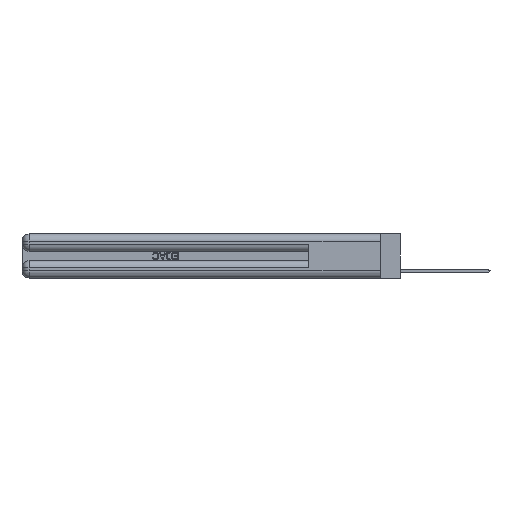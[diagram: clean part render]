
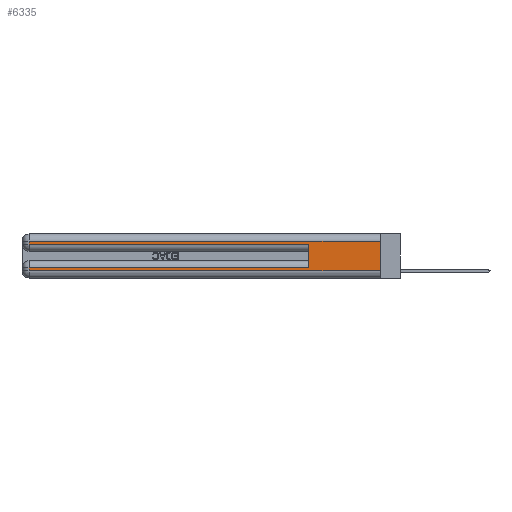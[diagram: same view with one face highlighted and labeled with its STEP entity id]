
A CAD part, left-side view. The second image highlights one B-rep face of the part: STEP entity #6335.
In plain terms, the highlighted planar face has unit normal (-1, 0, 0).
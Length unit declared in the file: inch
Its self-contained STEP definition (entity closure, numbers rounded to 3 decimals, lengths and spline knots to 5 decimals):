
#159 = EDGE_CURVE ( 'NONE', #7432, #27323, #20587, .T. ) ;
#514 = EDGE_CURVE ( 'NONE', #9815, #19662, #22352, .T. ) ;
#802 = VECTOR ( 'NONE', #28510, 39.37008 ) ;
#811 = CARTESIAN_POINT ( 'NONE',  ( 0., 2.94, 0.085 ) ) ;
#1375 = VERTEX_POINT ( 'NONE', #15266 ) ;
#1476 = CARTESIAN_POINT ( 'NONE',  ( 0., 0., 0.37 ) ) ;
#2492 = EDGE_CURVE ( 'NONE', #27323, #23398, #21660, .T. ) ;
#3552 = EDGE_CURVE ( 'NONE', #7432, #4708, #16799, .T. ) ;
#3866 = CARTESIAN_POINT ( 'NONE',  ( 0., 0., 0.06 ) ) ;
#3912 = CARTESIAN_POINT ( 'NONE',  ( 0., 0., 0.285 ) ) ;
#4686 = CARTESIAN_POINT ( 'NONE',  ( 0., 0., 0.31 ) ) ;
#4708 = VERTEX_POINT ( 'NONE', #11739 ) ;
#5120 = DIRECTION ( 'NONE',  ( 0., 1., 0. ) ) ;
#6276 = CARTESIAN_POINT ( 'NONE',  ( 0., 2.94, 0.31 ) ) ;
#6335 = ADVANCED_FACE ( 'NONE', ( #12847 ), #21866, .F. ) ;
#6800 = DIRECTION ( 'NONE',  ( 0., 0., -1. ) ) ;
#7001 = DIRECTION ( 'NONE',  ( 0., 1., 0. ) ) ;
#7432 = VERTEX_POINT ( 'NONE', #15799 ) ;
#7585 = VECTOR ( 'NONE', #6800, 39.37008 ) ;
#8403 = DIRECTION ( 'NONE',  ( 0., 0., -1. ) ) ;
#9815 = VERTEX_POINT ( 'NONE', #6276 ) ;
#10584 = LINE ( 'NONE', #3912, #23167 ) ;
#11206 = LINE ( 'NONE', #29340, #7585 ) ;
#11263 = ORIENTED_EDGE ( 'NONE', *, *, #159, .T. ) ;
#11739 = CARTESIAN_POINT ( 'NONE',  ( 0., 0.6, 0.285 ) ) ;
#11810 = CARTESIAN_POINT ( 'NONE',  ( 0., 2.94, 0.06 ) ) ;
#12237 = DIRECTION ( 'NONE',  ( 0., 0., 1. ) ) ;
#12847 = FACE_OUTER_BOUND ( 'NONE', #18352, .T. ) ;
#13469 = DIRECTION ( 'NONE',  ( 0., 0., -1. ) ) ;
#14163 = ORIENTED_EDGE ( 'NONE', *, *, #514, .T. ) ;
#14460 = ORIENTED_EDGE ( 'NONE', *, *, #27153, .T. ) ;
#14828 = AXIS2_PLACEMENT_3D ( 'NONE', #1476, #28695, #8403 ) ;
#14890 = VECTOR ( 'NONE', #7001, 39.37008 ) ;
#15266 = CARTESIAN_POINT ( 'NONE',  ( 0., 0., 0.06 ) ) ;
#15279 = CARTESIAN_POINT ( 'NONE',  ( 0., 0., 0.31 ) ) ;
#15638 = VERTEX_POINT ( 'NONE', #15279 ) ;
#15799 = CARTESIAN_POINT ( 'NONE',  ( 0., 0.6, 0.085 ) ) ;
#16082 = LINE ( 'NONE', #4686, #26034 ) ;
#16462 = DIRECTION ( 'NONE',  ( 0., 0., -1. ) ) ;
#16799 = LINE ( 'NONE', #19468, #29404 ) ;
#18352 = EDGE_LOOP ( 'NONE', ( #27959, #18497, #14163, #23790, #19272, #11263, #19184, #14460 ) ) ;
#18497 = ORIENTED_EDGE ( 'NONE', *, *, #29265, .T. ) ;
#19184 = ORIENTED_EDGE ( 'NONE', *, *, #2492, .T. ) ;
#19272 = ORIENTED_EDGE ( 'NONE', *, *, #3552, .F. ) ;
#19468 = CARTESIAN_POINT ( 'NONE',  ( 0., 0.6, 0.145 ) ) ;
#19662 = VERTEX_POINT ( 'NONE', #27298 ) ;
#19824 = DIRECTION ( 'NONE',  ( 0., -1., 0. ) ) ;
#20587 = LINE ( 'NONE', #27309, #14890 ) ;
#21277 = VECTOR ( 'NONE', #16462, 39.37008 ) ;
#21660 = LINE ( 'NONE', #27950, #21277 ) ;
#21866 = PLANE ( 'NONE',  #14828 ) ;
#22352 = LINE ( 'NONE', #22502, #25942 ) ;
#22502 = CARTESIAN_POINT ( 'NONE',  ( 0., 2.94, 0.37 ) ) ;
#23167 = VECTOR ( 'NONE', #19824, 39.37008 ) ;
#23398 = VERTEX_POINT ( 'NONE', #11810 ) ;
#23790 = ORIENTED_EDGE ( 'NONE', *, *, #27687, .T. ) ;
#24380 = LINE ( 'NONE', #3866, #802 ) ;
#25942 = VECTOR ( 'NONE', #13469, 39.37008 ) ;
#26034 = VECTOR ( 'NONE', #5120, 39.37008 ) ;
#27153 = EDGE_CURVE ( 'NONE', #23398, #1375, #24380, .T. ) ;
#27298 = CARTESIAN_POINT ( 'NONE',  ( 0., 2.94, 0.285 ) ) ;
#27309 = CARTESIAN_POINT ( 'NONE',  ( 0., 0., 0.085 ) ) ;
#27323 = VERTEX_POINT ( 'NONE', #811 ) ;
#27449 = EDGE_CURVE ( 'NONE', #15638, #1375, #11206, .T. ) ;
#27687 = EDGE_CURVE ( 'NONE', #19662, #4708, #10584, .T. ) ;
#27950 = CARTESIAN_POINT ( 'NONE',  ( 0., 2.94, 0.37 ) ) ;
#27959 = ORIENTED_EDGE ( 'NONE', *, *, #27449, .F. ) ;
#28510 = DIRECTION ( 'NONE',  ( 0., -1., 0. ) ) ;
#28695 = DIRECTION ( 'NONE',  ( 1., 0., 0. ) ) ;
#29265 = EDGE_CURVE ( 'NONE', #15638, #9815, #16082, .T. ) ;
#29340 = CARTESIAN_POINT ( 'NONE',  ( 0., 0., 0.37 ) ) ;
#29404 = VECTOR ( 'NONE', #12237, 39.37008 ) ;
